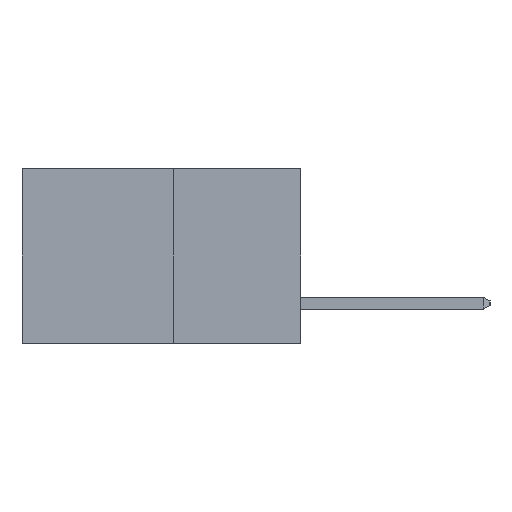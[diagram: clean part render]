
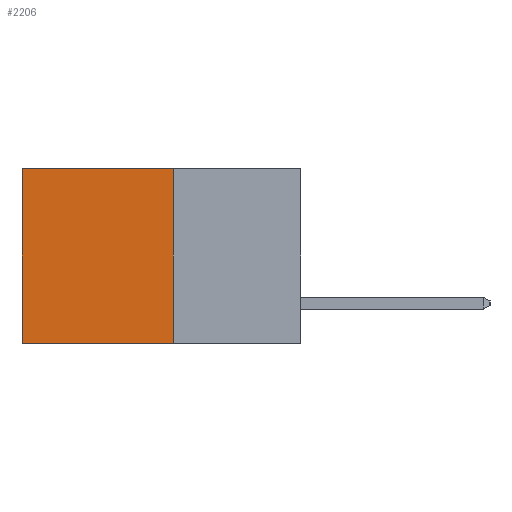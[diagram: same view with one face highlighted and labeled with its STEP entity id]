
A CAD part, left-side view. The second image highlights one B-rep face of the part: STEP entity #2206.
In plain terms, the highlighted planar face has unit normal (-1, 0, 0).
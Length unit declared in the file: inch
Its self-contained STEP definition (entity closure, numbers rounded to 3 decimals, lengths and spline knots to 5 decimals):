
#74 = VECTOR ( 'NONE', #3742, 39.37008 ) ;
#385 = FACE_OUTER_BOUND ( 'NONE', #5824, .T. ) ;
#430 = LINE ( 'NONE', #6466, #7827 ) ;
#448 = DIRECTION ( 'NONE',  ( 1., 0., 0. ) ) ;
#1719 = DIRECTION ( 'NONE',  ( 0., 0., -1. ) ) ;
#1759 = VERTEX_POINT ( 'NONE', #6599 ) ;
#1974 = VECTOR ( 'NONE', #9000, 39.37008 ) ;
#2206 = ADVANCED_FACE ( 'NONE', ( #385 ), #8616, .F. ) ;
#3289 = EDGE_CURVE ( 'NONE', #6405, #4918, #5068, .T. ) ;
#3389 = CARTESIAN_POINT ( 'NONE',  ( 0.277, 0.59, -0.37 ) ) ;
#3393 = CARTESIAN_POINT ( 'NONE',  ( 0.277, 0.27, -0.37 ) ) ;
#3446 = EDGE_CURVE ( 'NONE', #1759, #6405, #6068, .T. ) ;
#3742 = DIRECTION ( 'NONE',  ( 0., 1., 0. ) ) ;
#3779 = LINE ( 'NONE', #7222, #74 ) ;
#4307 = AXIS2_PLACEMENT_3D ( 'NONE', #8530, #448, #1719 ) ;
#4521 = ORIENTED_EDGE ( 'NONE', *, *, #3289, .F. ) ;
#4812 = CARTESIAN_POINT ( 'NONE',  ( 0.277, 0.27, -0.37 ) ) ;
#4831 = CARTESIAN_POINT ( 'NONE',  ( 0.277, 0.27, -0.37 ) ) ;
#4918 = VERTEX_POINT ( 'NONE', #3389 ) ;
#5068 = LINE ( 'NONE', #4831, #6915 ) ;
#5238 = ORIENTED_EDGE ( 'NONE', *, *, #3446, .F. ) ;
#5674 = ORIENTED_EDGE ( 'NONE', *, *, #6993, .T. ) ;
#5824 = EDGE_LOOP ( 'NONE', ( #5674, #4521, #5238, #8785 ) ) ;
#6068 = LINE ( 'NONE', #4812, #1974 ) ;
#6383 = DIRECTION ( 'NONE',  ( 0., 0., -1. ) ) ;
#6405 = VERTEX_POINT ( 'NONE', #3393 ) ;
#6466 = CARTESIAN_POINT ( 'NONE',  ( 0.277, 0.59, -0.37 ) ) ;
#6599 = CARTESIAN_POINT ( 'NONE',  ( 0.277, 0.27, 0. ) ) ;
#6915 = VECTOR ( 'NONE', #8514, 39.37008 ) ;
#6993 = EDGE_CURVE ( 'NONE', #8255, #4918, #430, .T. ) ;
#7222 = CARTESIAN_POINT ( 'NONE',  ( 0.277, 0.27, 0. ) ) ;
#7827 = VECTOR ( 'NONE', #6383, 39.37008 ) ;
#8255 = VERTEX_POINT ( 'NONE', #9143 ) ;
#8409 = EDGE_CURVE ( 'NONE', #1759, #8255, #3779, .T. ) ;
#8514 = DIRECTION ( 'NONE',  ( 0., 1., 0. ) ) ;
#8530 = CARTESIAN_POINT ( 'NONE',  ( 0.277, 0.27, -0.37 ) ) ;
#8616 = PLANE ( 'NONE',  #4307 ) ;
#8785 = ORIENTED_EDGE ( 'NONE', *, *, #8409, .T. ) ;
#9000 = DIRECTION ( 'NONE',  ( 0., 0., -1. ) ) ;
#9143 = CARTESIAN_POINT ( 'NONE',  ( 0.277, 0.59, 0. ) ) ;
